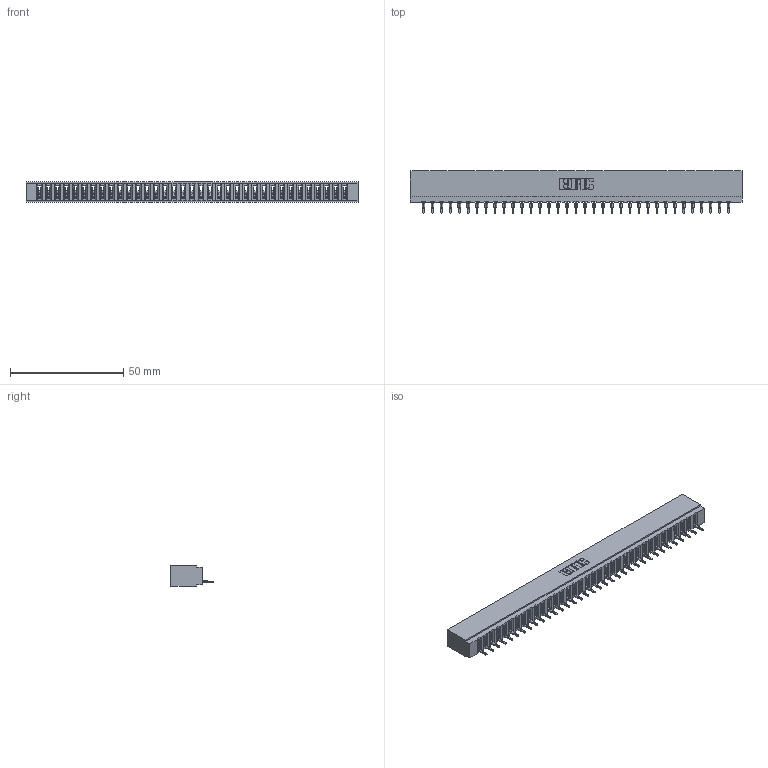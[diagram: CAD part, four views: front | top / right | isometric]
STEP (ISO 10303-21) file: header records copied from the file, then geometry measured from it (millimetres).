
FILE_DESCRIPTION (( 'STEP AP203' ), '1' );
FILE_NAME ('717-035-520-101.STEP', '2026-02-20T21:43:49', ( '' ), ( '' ), 'SwSTEP 2.0', 'SolidWorks 2023', '' );
FILE_SCHEMA (( 'CONFIG_CONTROL_DESIGN' ));
Length unit declared in the file: millimetre
Products named in the file (3): 717-035-520-101; 717 Part_Insulator Option - 06; 745-292-001_520
Assembly tree (36 placements, depth 2):
  717-035-520-101
    717 Part_Insulator Option - 06
    745-292-001_520  x35
Bounding box: 146.56 x 18.78 x 8.89 mm (x, y, z)
Volume: 12355.8 mm3; surface area: 17034.2 mm2
Topology: 36 solids, 36 shells, 4049 faces, 11136 edges, 7026 vertices
Faces by surface type: plane 2434, cylinder 705, bspline 700, torus 210
Entity records: 59845 total; most frequent: CARTESIAN_POINT 11052, ORIENTED_EDGE 10508, DIRECTION 9110, EDGE_CURVE 5254, LINE 4862, VECTOR 4862, VERTEX_POINT 3354, AXIS2_PLACEMENT_3D 2124
